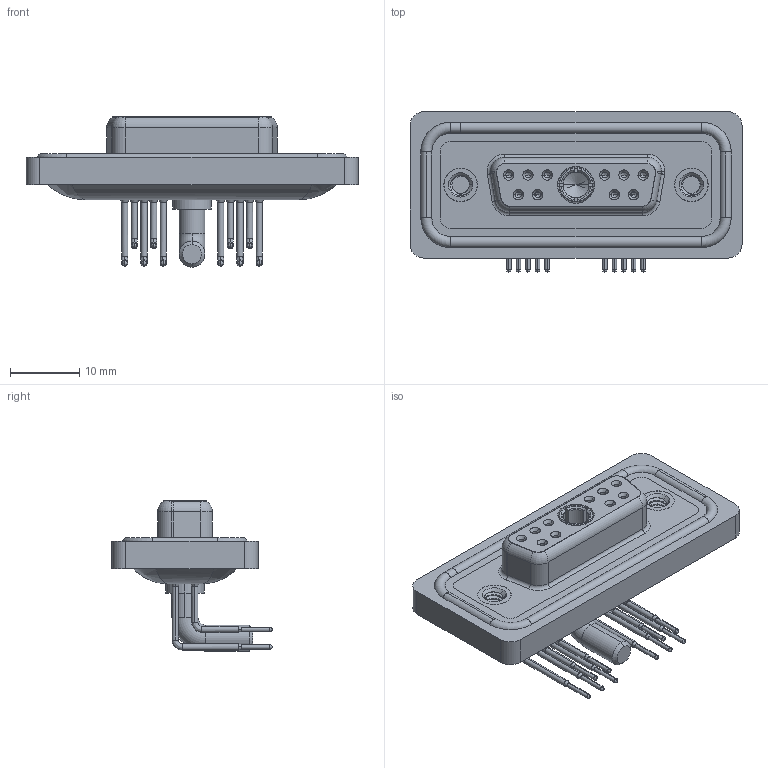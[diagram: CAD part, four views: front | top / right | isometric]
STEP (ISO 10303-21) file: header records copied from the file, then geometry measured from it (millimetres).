
FILE_DESCRIPTION (( 'STEP AP203' ), '1' );
FILE_NAME ('630W11W1640-4NA.STEP', '2024-04-12T00:13:32', ( '' ), ( '' ), 'SwSTEP 2.0', 'SolidWorks 2023', '' );
FILE_SCHEMA (( 'CONFIG_CONTROL_DESIGN' ));
Length unit declared in the file: millimetre
Products named in the file (9): 630Combo Housing_11W1; 630Combo Shell Rear_15 Contacts; 630W11W1640-4NA; 630Combo Contact Row 1_50 Contacts; 630Combo Waterproof Housing_15 Contacts; 630Combo Shell Front_15 Contacts; 630Combo Contact Row 2_50 Contacts; Power Socket_40A RA; 630Combo Threaded Rivet_A
Assembly tree (17 placements, depth 2):
  630W11W1640-4NA
    630Combo Housing_11W1
    630Combo Shell Front_15 Contacts
    630Combo Shell Rear_15 Contacts
    630Combo Threaded Rivet_A  x2
    Power Socket_40A RA
    630Combo Contact Row 1_50 Contacts  x6
    630Combo Contact Row 2_50 Contacts  x4
    630Combo Waterproof Housing_15 Contacts
Bounding box: 47.9 x 23.12 x 21.68 mm (x, y, z)
Volume: 6283 mm3; surface area: 10517.6 mm2
Topology: 19 solids, 19 shells, 988 faces, 2499 edges, 1573 vertices
Faces by surface type: cylinder 441, plane 284, cone 135, torus 77, bspline 51
Entity records: 22205 total; most frequent: CARTESIAN_POINT 5594, DIRECTION 3455, ORIENTED_EDGE 3106, EDGE_CURVE 1553, AXIS2_PLACEMENT_3D 1407, VERTEX_POINT 989, CIRCLE 765, EDGE_LOOP 730
